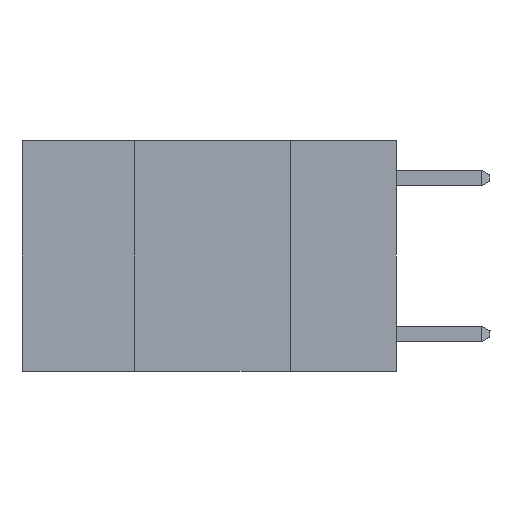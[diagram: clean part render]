
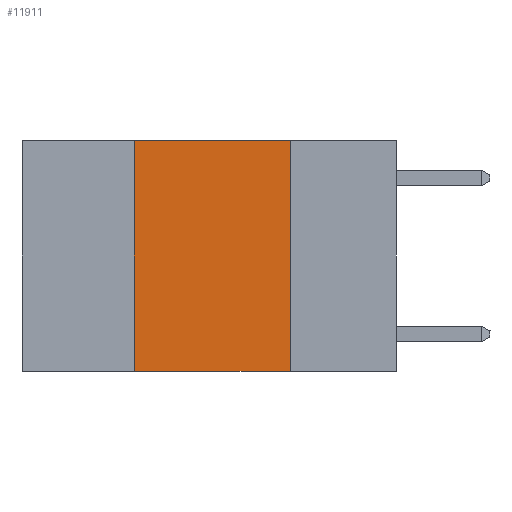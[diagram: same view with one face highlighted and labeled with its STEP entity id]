
A CAD part, left-side view. The second image highlights one B-rep face of the part: STEP entity #11911.
In plain terms, the highlighted planar face has unit normal (-1, 0, 0).
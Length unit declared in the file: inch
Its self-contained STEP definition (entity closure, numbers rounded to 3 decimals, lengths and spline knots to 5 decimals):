
#940 = EDGE_CURVE ( 'NONE', #3398, #24056, #23291, .T. ) ;
#1139 = LINE ( 'NONE', #26082, #11547 ) ;
#1703 = EDGE_LOOP ( 'NONE', ( #6194, #6326, #6455, #7031 ) ) ;
#1794 = CARTESIAN_POINT ( 'NONE',  ( 0., 0.6, 0. ) ) ;
#2984 = CARTESIAN_POINT ( 'NONE',  ( 0., 0.42, -0.37 ) ) ;
#3398 = VERTEX_POINT ( 'NONE', #2984 ) ;
#3929 = DIRECTION ( 'NONE',  ( 0., 0., -1. ) ) ;
#4552 = AXIS2_PLACEMENT_3D ( 'NONE', #1794, #17282, #3929 ) ;
#5174 = VERTEX_POINT ( 'NONE', #8461 ) ;
#6194 = ORIENTED_EDGE ( 'NONE', *, *, #20717, .F. ) ;
#6326 = ORIENTED_EDGE ( 'NONE', *, *, #13081, .F. ) ;
#6455 = ORIENTED_EDGE ( 'NONE', *, *, #940, .F. ) ;
#7031 = ORIENTED_EDGE ( 'NONE', *, *, #19896, .T. ) ;
#7950 = DIRECTION ( 'NONE',  ( 0., -1., 0. ) ) ;
#8461 = CARTESIAN_POINT ( 'NONE',  ( 0., 0.17, 0. ) ) ;
#11442 = DIRECTION ( 'NONE',  ( 0., -1., 0. ) ) ;
#11547 = VECTOR ( 'NONE', #11442, 39.37008 ) ;
#11911 = ADVANCED_FACE ( 'NONE', ( #23594 ), #21331, .F. ) ;
#12558 = CARTESIAN_POINT ( 'NONE',  ( 0., 0.6, -0.37 ) ) ;
#13081 = EDGE_CURVE ( 'NONE', #24056, #5174, #1139, .T. ) ;
#13512 = CARTESIAN_POINT ( 'NONE',  ( 0., 0.17, -0.37 ) ) ;
#14121 = LINE ( 'NONE', #25449, #19060 ) ;
#17282 = DIRECTION ( 'NONE',  ( 1., 0., 0. ) ) ;
#19060 = VECTOR ( 'NONE', #19331, 39.37008 ) ;
#19331 = DIRECTION ( 'NONE',  ( 0., 0., -1. ) ) ;
#19896 = EDGE_CURVE ( 'NONE', #3398, #22617, #24833, .T. ) ;
#20409 = CARTESIAN_POINT ( 'NONE',  ( 0., 0.42, 0. ) ) ;
#20717 = EDGE_CURVE ( 'NONE', #5174, #22617, #14121, .T. ) ;
#21331 = PLANE ( 'NONE',  #4552 ) ;
#22617 = VERTEX_POINT ( 'NONE', #13512 ) ;
#22959 = CARTESIAN_POINT ( 'NONE',  ( 0., 0.42, 0. ) ) ;
#23239 = VECTOR ( 'NONE', #24302, 39.37008 ) ;
#23291 = LINE ( 'NONE', #20409, #23239 ) ;
#23594 = FACE_OUTER_BOUND ( 'NONE', #1703, .T. ) ;
#24056 = VERTEX_POINT ( 'NONE', #22959 ) ;
#24193 = VECTOR ( 'NONE', #7950, 39.37008 ) ;
#24302 = DIRECTION ( 'NONE',  ( 0., 0., 1. ) ) ;
#24833 = LINE ( 'NONE', #12558, #24193 ) ;
#25449 = CARTESIAN_POINT ( 'NONE',  ( 0., 0.17, 0. ) ) ;
#26082 = CARTESIAN_POINT ( 'NONE',  ( 0., 0.6, 0. ) ) ;
